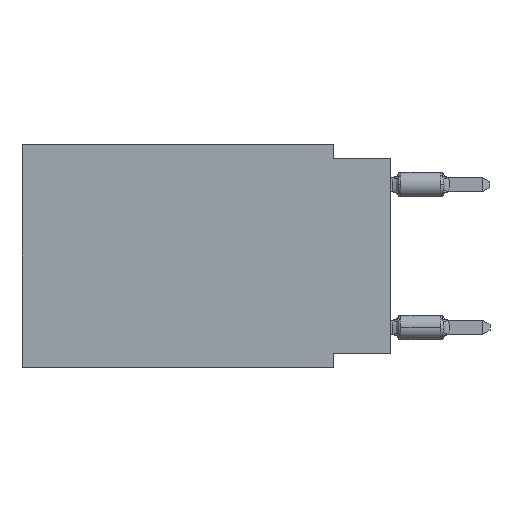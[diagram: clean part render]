
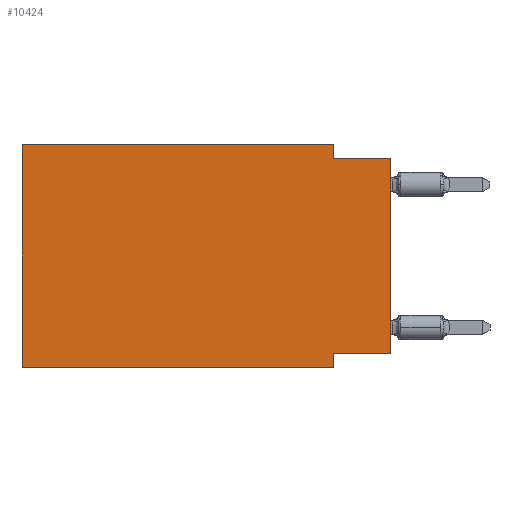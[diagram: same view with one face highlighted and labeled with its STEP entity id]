
A CAD part, left-side view. The second image highlights one B-rep face of the part: STEP entity #10424.
In plain terms, the highlighted planar face has unit normal (-1, 0, 0).
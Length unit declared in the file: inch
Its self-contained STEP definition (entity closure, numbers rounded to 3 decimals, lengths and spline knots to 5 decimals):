
#3168 = VERTEX_POINT ( 'NONE', #7035 ) ;
#3493 = DIRECTION ( 'NONE',  ( 0., 0., -1. ) ) ;
#4529 = CARTESIAN_POINT ( 'NONE',  ( 0., 0., -0.025 ) ) ;
#4543 = VERTEX_POINT ( 'NONE', #4529 ) ;
#4628 = CARTESIAN_POINT ( 'NONE',  ( 0., 0.645, -0.39 ) ) ;
#5714 = LINE ( 'NONE', #13446, #34836 ) ;
#6384 = VECTOR ( 'NONE', #10191, 39.37008 ) ;
#6780 = CARTESIAN_POINT ( 'NONE',  ( 0., 0., -0.365 ) ) ;
#6998 = CARTESIAN_POINT ( 'NONE',  ( 0., 0.645, -0.39 ) ) ;
#7035 = CARTESIAN_POINT ( 'NONE',  ( 0., 0.1, -0.025 ) ) ;
#8601 = AXIS2_PLACEMENT_3D ( 'NONE', #30492, #28150, #3493 ) ;
#8875 = LINE ( 'NONE', #9415, #31377 ) ;
#8891 = VERTEX_POINT ( 'NONE', #25622 ) ;
#9415 = CARTESIAN_POINT ( 'NONE',  ( 0., 0.1, -0.39 ) ) ;
#9661 = CARTESIAN_POINT ( 'NONE',  ( 0., 0., -0.365 ) ) ;
#10191 = DIRECTION ( 'NONE',  ( 0., -1., 0. ) ) ;
#10424 = ADVANCED_FACE ( 'NONE', ( #19520 ), #30828, .F. ) ;
#11446 = ORIENTED_EDGE ( 'NONE', *, *, #25933, .F. ) ;
#11727 = VERTEX_POINT ( 'NONE', #25196 ) ;
#13274 = ORIENTED_EDGE ( 'NONE', *, *, #30465, .F. ) ;
#13446 = CARTESIAN_POINT ( 'NONE',  ( 0., 0., -0.025 ) ) ;
#13502 = EDGE_CURVE ( 'NONE', #14622, #11727, #23320, .T. ) ;
#14242 = EDGE_CURVE ( 'NONE', #22523, #3168, #29319, .T. ) ;
#14412 = VECTOR ( 'NONE', #27022, 39.37008 ) ;
#14622 = VERTEX_POINT ( 'NONE', #9661 ) ;
#15168 = EDGE_LOOP ( 'NONE', ( #35499, #13274, #35288, #11446, #30041, #27926, #32194, #29359 ) ) ;
#16318 = LINE ( 'NONE', #19374, #23838 ) ;
#16785 = DIRECTION ( 'NONE',  ( 0., 0., 1. ) ) ;
#16928 = EDGE_CURVE ( 'NONE', #11727, #8891, #8875, .T. ) ;
#17149 = CARTESIAN_POINT ( 'NONE',  ( 0., 0., 0. ) ) ;
#17764 = EDGE_CURVE ( 'NONE', #27462, #21657, #16318, .T. ) ;
#18264 = VECTOR ( 'NONE', #16785, 39.37008 ) ;
#19374 = CARTESIAN_POINT ( 'NONE',  ( 0., 0.645, 0. ) ) ;
#19520 = FACE_OUTER_BOUND ( 'NONE', #15168, .T. ) ;
#21029 = CARTESIAN_POINT ( 'NONE',  ( 0., 0.1, 0. ) ) ;
#21374 = CARTESIAN_POINT ( 'NONE',  ( 0., 0.1, 0. ) ) ;
#21459 = CARTESIAN_POINT ( 'NONE',  ( 0., 0.645, 0. ) ) ;
#21657 = VERTEX_POINT ( 'NONE', #21459 ) ;
#22523 = VERTEX_POINT ( 'NONE', #21374 ) ;
#23320 = LINE ( 'NONE', #6780, #27972 ) ;
#23838 = VECTOR ( 'NONE', #30340, 39.37008 ) ;
#24306 = CARTESIAN_POINT ( 'NONE',  ( 0., 0.645, 0. ) ) ;
#25196 = CARTESIAN_POINT ( 'NONE',  ( 0., 0.1, -0.365 ) ) ;
#25622 = CARTESIAN_POINT ( 'NONE',  ( 0., 0.1, -0.39 ) ) ;
#25930 = DIRECTION ( 'NONE',  ( 0., 0., -1. ) ) ;
#25933 = EDGE_CURVE ( 'NONE', #21657, #22523, #32240, .T. ) ;
#26193 = EDGE_CURVE ( 'NONE', #27462, #8891, #29278, .T. ) ;
#27022 = DIRECTION ( 'NONE',  ( 0., -1., 0. ) ) ;
#27462 = VERTEX_POINT ( 'NONE', #6998 ) ;
#27576 = VECTOR ( 'NONE', #25930, 39.37008 ) ;
#27926 = ORIENTED_EDGE ( 'NONE', *, *, #26193, .T. ) ;
#27972 = VECTOR ( 'NONE', #33969, 39.37008 ) ;
#28150 = DIRECTION ( 'NONE',  ( 1., 0., 0. ) ) ;
#29278 = LINE ( 'NONE', #4628, #6384 ) ;
#29319 = LINE ( 'NONE', #21029, #27576 ) ;
#29359 = ORIENTED_EDGE ( 'NONE', *, *, #13502, .F. ) ;
#30041 = ORIENTED_EDGE ( 'NONE', *, *, #17764, .F. ) ;
#30340 = DIRECTION ( 'NONE',  ( 0., 0., 1. ) ) ;
#30465 = EDGE_CURVE ( 'NONE', #3168, #4543, #5714, .T. ) ;
#30492 = CARTESIAN_POINT ( 'NONE',  ( 0., 0.645, 0. ) ) ;
#30619 = LINE ( 'NONE', #17149, #18264 ) ;
#30828 = PLANE ( 'NONE',  #8601 ) ;
#31377 = VECTOR ( 'NONE', #33722, 39.37008 ) ;
#32194 = ORIENTED_EDGE ( 'NONE', *, *, #16928, .F. ) ;
#32201 = EDGE_CURVE ( 'NONE', #14622, #4543, #30619, .T. ) ;
#32240 = LINE ( 'NONE', #24306, #14412 ) ;
#33722 = DIRECTION ( 'NONE',  ( 0., 0., -1. ) ) ;
#33969 = DIRECTION ( 'NONE',  ( 0., 1., 0. ) ) ;
#34836 = VECTOR ( 'NONE', #35241, 39.37008 ) ;
#35241 = DIRECTION ( 'NONE',  ( 0., -1., 0. ) ) ;
#35288 = ORIENTED_EDGE ( 'NONE', *, *, #14242, .F. ) ;
#35499 = ORIENTED_EDGE ( 'NONE', *, *, #32201, .T. ) ;
